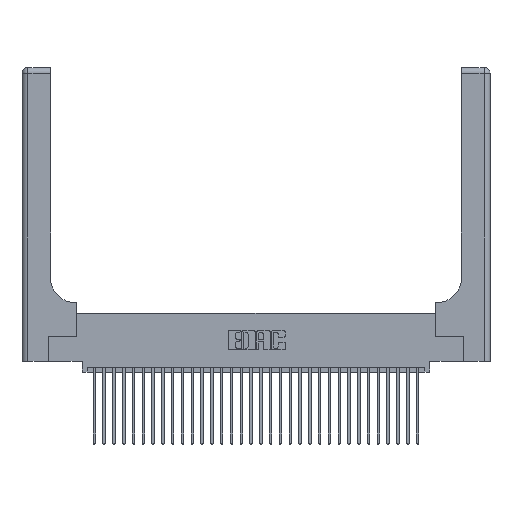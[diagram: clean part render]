
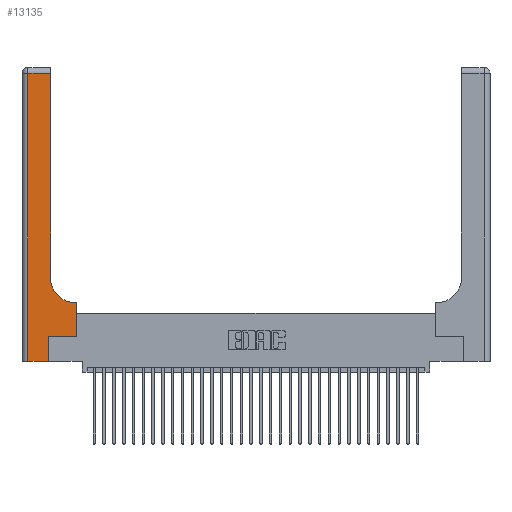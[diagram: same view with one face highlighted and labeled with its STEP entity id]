
A CAD part, top view. The second image highlights one B-rep face of the part: STEP entity #13135.
In plain terms, the highlighted planar face has unit normal (0, 0, 1).
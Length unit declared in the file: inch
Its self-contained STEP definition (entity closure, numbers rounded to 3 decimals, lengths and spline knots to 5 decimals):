
#441 = VECTOR ( 'NONE', #31431, 39.37008 ) ;
#453 = LINE ( 'NONE', #18202, #27728 ) ;
#1572 = DIRECTION ( 'NONE',  ( -1., 0., 0. ) ) ;
#1777 = CARTESIAN_POINT ( 'NONE',  ( 0.5415, 0.85, 0.37 ) ) ;
#2119 = CARTESIAN_POINT ( 'NONE',  ( 0.269, 0., 0.37 ) ) ;
#2313 = EDGE_CURVE ( 'NONE', #12335, #9409, #26899, .T. ) ;
#2727 = DIRECTION ( 'NONE',  ( 0., 1., 0. ) ) ;
#2773 = ORIENTED_EDGE ( 'NONE', *, *, #2313, .T. ) ;
#3136 = DIRECTION ( 'NONE',  ( 0., 0., -1. ) ) ;
#4318 = ORIENTED_EDGE ( 'NONE', *, *, #13872, .T. ) ;
#4455 = VERTEX_POINT ( 'NONE', #11645 ) ;
#4819 = EDGE_CURVE ( 'NONE', #12064, #8981, #21992, .T. ) ;
#5520 = DIRECTION ( 'NONE',  ( 0., 1., 0. ) ) ;
#6168 = CARTESIAN_POINT ( 'NONE',  ( 0.06, 3., 0.37 ) ) ;
#8092 = CIRCLE ( 'NONE', #29795, 0.25 ) ;
#8181 = VECTOR ( 'NONE', #2727, 39.37008 ) ;
#8324 = EDGE_CURVE ( 'NONE', #22964, #12335, #8480, .T. ) ;
#8480 = LINE ( 'NONE', #6168, #441 ) ;
#8981 = VERTEX_POINT ( 'NONE', #18591 ) ;
#9390 = DIRECTION ( 'NONE',  ( 1., 0., 0. ) ) ;
#9409 = VERTEX_POINT ( 'NONE', #2119 ) ;
#9897 = VERTEX_POINT ( 'NONE', #23696 ) ;
#11645 = CARTESIAN_POINT ( 'NONE',  ( 0.2915, 2.94, 0.37 ) ) ;
#11830 = DIRECTION ( 'NONE',  ( 0., 1., 0. ) ) ;
#11896 = CARTESIAN_POINT ( 'NONE',  ( 0., 3., 0.37 ) ) ;
#11900 = CARTESIAN_POINT ( 'NONE',  ( 0.2915, 0.6, 0.37 ) ) ;
#12064 = VERTEX_POINT ( 'NONE', #17192 ) ;
#12335 = VERTEX_POINT ( 'NONE', #31756 ) ;
#12456 = DIRECTION ( 'NONE',  ( 0., 0., -1. ) ) ;
#13027 = ORIENTED_EDGE ( 'NONE', *, *, #18393, .T. ) ;
#13135 = ADVANCED_FACE ( 'NONE', ( #20796 ), #23643, .F. ) ;
#13872 = EDGE_CURVE ( 'NONE', #31512, #12064, #22403, .T. ) ;
#15000 = LINE ( 'NONE', #30789, #8181 ) ;
#15042 = VERTEX_POINT ( 'NONE', #28631 ) ;
#15971 = EDGE_CURVE ( 'NONE', #15042, #4455, #29027, .T. ) ;
#16838 = AXIS2_PLACEMENT_3D ( 'NONE', #11896, #3136, #20120 ) ;
#17192 = CARTESIAN_POINT ( 'NONE',  ( 0.5585, 0.25, 0.37 ) ) ;
#17661 = LINE ( 'NONE', #11900, #20085 ) ;
#18202 = CARTESIAN_POINT ( 'NONE',  ( 0., 2.94, 0.37 ) ) ;
#18267 = EDGE_CURVE ( 'NONE', #9897, #15042, #8092, .T. ) ;
#18393 = EDGE_CURVE ( 'NONE', #4455, #22964, #453, .T. ) ;
#18591 = CARTESIAN_POINT ( 'NONE',  ( 0.5585, 0.6, 0.37 ) ) ;
#19494 = ORIENTED_EDGE ( 'NONE', *, *, #18267, .T. ) ;
#19716 = VECTOR ( 'NONE', #32359, 39.37008 ) ;
#19777 = EDGE_LOOP ( 'NONE', ( #23604, #13027, #31432, #2773, #29001, #4318, #30835, #21240, #19494 ) ) ;
#20085 = VECTOR ( 'NONE', #1572, 39.37008 ) ;
#20120 = DIRECTION ( 'NONE',  ( -1., 0., 0. ) ) ;
#20796 = FACE_OUTER_BOUND ( 'NONE', #19777, .T. ) ;
#20961 = CARTESIAN_POINT ( 'NONE',  ( 0.2915, 3., 0.37 ) ) ;
#21240 = ORIENTED_EDGE ( 'NONE', *, *, #27933, .T. ) ;
#21418 = VECTOR ( 'NONE', #5520, 39.37008 ) ;
#21916 = CARTESIAN_POINT ( 'NONE',  ( 0.269, 0.25, 0.37 ) ) ;
#21992 = LINE ( 'NONE', #29626, #23914 ) ;
#22403 = LINE ( 'NONE', #21916, #28756 ) ;
#22964 = VERTEX_POINT ( 'NONE', #28162 ) ;
#23456 = DIRECTION ( 'NONE',  ( -1., 0., 0. ) ) ;
#23549 = EDGE_CURVE ( 'NONE', #9409, #31512, #15000, .T. ) ;
#23604 = ORIENTED_EDGE ( 'NONE', *, *, #15971, .T. ) ;
#23643 = PLANE ( 'NONE',  #16838 ) ;
#23696 = CARTESIAN_POINT ( 'NONE',  ( 0.5415, 0.6, 0.37 ) ) ;
#23914 = VECTOR ( 'NONE', #11830, 39.37008 ) ;
#26507 = CARTESIAN_POINT ( 'NONE',  ( 0.269, 0.25, 0.37 ) ) ;
#26899 = LINE ( 'NONE', #31473, #19716 ) ;
#27728 = VECTOR ( 'NONE', #23456, 39.37008 ) ;
#27933 = EDGE_CURVE ( 'NONE', #8981, #9897, #17661, .T. ) ;
#28162 = CARTESIAN_POINT ( 'NONE',  ( 0.06, 2.94, 0.37 ) ) ;
#28631 = CARTESIAN_POINT ( 'NONE',  ( 0.2915, 0.85, 0.37 ) ) ;
#28756 = VECTOR ( 'NONE', #9390, 39.37008 ) ;
#29001 = ORIENTED_EDGE ( 'NONE', *, *, #23549, .T. ) ;
#29027 = LINE ( 'NONE', #20961, #21418 ) ;
#29626 = CARTESIAN_POINT ( 'NONE',  ( 0.5585, 0.25, 0.37 ) ) ;
#29795 = AXIS2_PLACEMENT_3D ( 'NONE', #1777, #12456, #30326 ) ;
#30326 = DIRECTION ( 'NONE',  ( 1., 0., 0. ) ) ;
#30789 = CARTESIAN_POINT ( 'NONE',  ( 0.269, 0., 0.37 ) ) ;
#30835 = ORIENTED_EDGE ( 'NONE', *, *, #4819, .T. ) ;
#31431 = DIRECTION ( 'NONE',  ( 0., -1., 0. ) ) ;
#31432 = ORIENTED_EDGE ( 'NONE', *, *, #8324, .T. ) ;
#31473 = CARTESIAN_POINT ( 'NONE',  ( 0., 0., 0.37 ) ) ;
#31512 = VERTEX_POINT ( 'NONE', #26507 ) ;
#31756 = CARTESIAN_POINT ( 'NONE',  ( 0.06, 0., 0.37 ) ) ;
#32359 = DIRECTION ( 'NONE',  ( 1., 0., 0. ) ) ;
